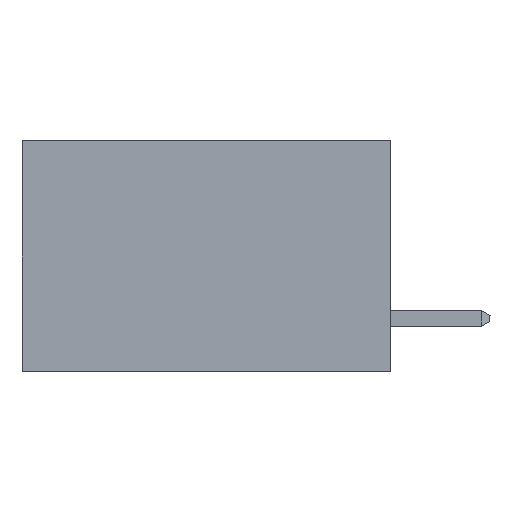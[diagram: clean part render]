
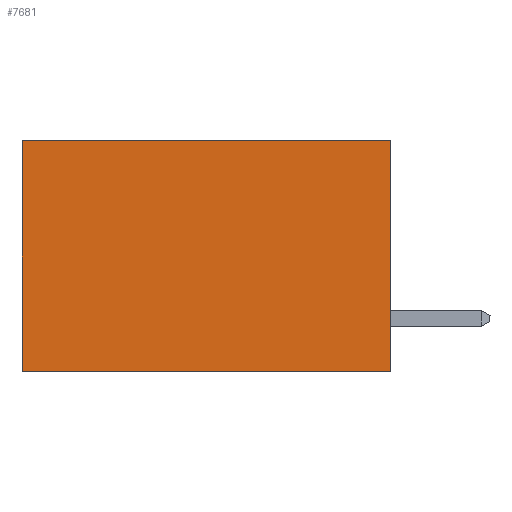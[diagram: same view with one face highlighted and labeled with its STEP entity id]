
A CAD part, left-side view. The second image highlights one B-rep face of the part: STEP entity #7681.
In plain terms, the highlighted planar face has unit normal (-1, 0, 0).
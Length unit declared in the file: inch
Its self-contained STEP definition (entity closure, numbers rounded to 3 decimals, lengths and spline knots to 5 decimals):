
#48 = VERTEX_POINT ( 'NONE', #3503 ) ;
#217 = EDGE_LOOP ( 'NONE', ( #9848, #3024, #9172, #4969 ) ) ;
#1018 = LINE ( 'NONE', #14257, #4410 ) ;
#1189 = VECTOR ( 'NONE', #17234, 39.37008 ) ;
#2662 = CARTESIAN_POINT ( 'NONE',  ( 0.277, 0., -0.37 ) ) ;
#3024 = ORIENTED_EDGE ( 'NONE', *, *, #17160, .F. ) ;
#3100 = PLANE ( 'NONE',  #17878 ) ;
#3503 = CARTESIAN_POINT ( 'NONE',  ( 0.277, 0., -0.37 ) ) ;
#4410 = VECTOR ( 'NONE', #12868, 39.37008 ) ;
#4926 = EDGE_CURVE ( 'NONE', #13044, #48, #6434, .T. ) ;
#4969 = ORIENTED_EDGE ( 'NONE', *, *, #12335, .T. ) ;
#5276 = DIRECTION ( 'NONE',  ( 1., 0., 0. ) ) ;
#5662 = DIRECTION ( 'NONE',  ( 0., 0., -1. ) ) ;
#5755 = VERTEX_POINT ( 'NONE', #6486 ) ;
#5853 = CARTESIAN_POINT ( 'NONE',  ( 0.277, 0.59, -0.37 ) ) ;
#6434 = LINE ( 'NONE', #15999, #16977 ) ;
#6486 = CARTESIAN_POINT ( 'NONE',  ( 0.277, 0.59, 0. ) ) ;
#7681 = ADVANCED_FACE ( 'NONE', ( #15599 ), #3100, .F. ) ;
#7962 = CARTESIAN_POINT ( 'NONE',  ( 0.277, 0., 0. ) ) ;
#8742 = LINE ( 'NONE', #15846, #1189 ) ;
#9172 = ORIENTED_EDGE ( 'NONE', *, *, #4926, .F. ) ;
#9261 = LINE ( 'NONE', #5853, #12484 ) ;
#9553 = CARTESIAN_POINT ( 'NONE',  ( 0.277, 0.59, -0.37 ) ) ;
#9848 = ORIENTED_EDGE ( 'NONE', *, *, #15859, .T. ) ;
#12335 = EDGE_CURVE ( 'NONE', #13044, #5755, #8742, .T. ) ;
#12484 = VECTOR ( 'NONE', #15510, 39.37008 ) ;
#12868 = DIRECTION ( 'NONE',  ( 0., 1., 0. ) ) ;
#13044 = VERTEX_POINT ( 'NONE', #7962 ) ;
#14257 = CARTESIAN_POINT ( 'NONE',  ( 0.277, 0., -0.37 ) ) ;
#14458 = VERTEX_POINT ( 'NONE', #9553 ) ;
#15510 = DIRECTION ( 'NONE',  ( 0., 0., -1. ) ) ;
#15599 = FACE_OUTER_BOUND ( 'NONE', #217, .T. ) ;
#15818 = DIRECTION ( 'NONE',  ( 0., 0., -1. ) ) ;
#15846 = CARTESIAN_POINT ( 'NONE',  ( 0.277, 0., 0. ) ) ;
#15859 = EDGE_CURVE ( 'NONE', #5755, #14458, #9261, .T. ) ;
#15999 = CARTESIAN_POINT ( 'NONE',  ( 0.277, 0., -0.37 ) ) ;
#16977 = VECTOR ( 'NONE', #15818, 39.37008 ) ;
#17160 = EDGE_CURVE ( 'NONE', #48, #14458, #1018, .T. ) ;
#17234 = DIRECTION ( 'NONE',  ( 0., 1., 0. ) ) ;
#17878 = AXIS2_PLACEMENT_3D ( 'NONE', #2662, #5276, #5662 ) ;
